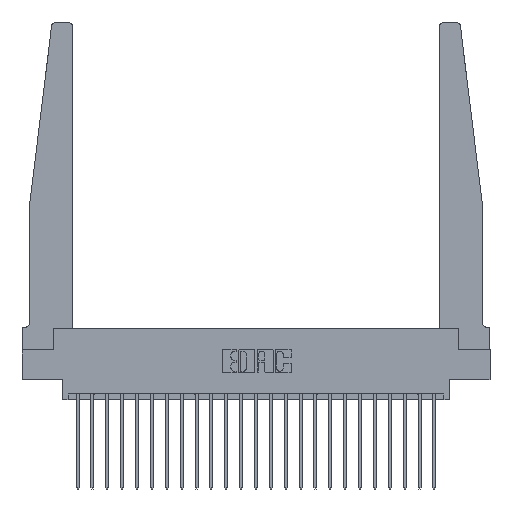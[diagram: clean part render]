
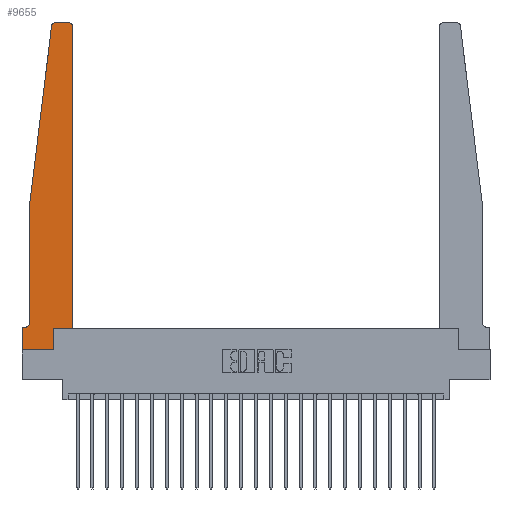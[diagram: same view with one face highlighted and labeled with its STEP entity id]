
A CAD part, top view. The second image highlights one B-rep face of the part: STEP entity #9655.
In plain terms, the highlighted planar face has unit normal (0, 0, 1).
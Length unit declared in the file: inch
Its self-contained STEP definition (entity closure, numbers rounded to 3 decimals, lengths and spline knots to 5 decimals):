
#130 = VERTEX_POINT ( 'NONE', #22104 ) ;
#207 = VERTEX_POINT ( 'NONE', #505 ) ;
#505 = CARTESIAN_POINT ( 'NONE',  ( 0.015, 0.1875, 0.37 ) ) ;
#706 = VERTEX_POINT ( 'NONE', #720 ) ;
#716 = CARTESIAN_POINT ( 'NONE',  ( 0., 0.1875, 0.37 ) ) ;
#720 = CARTESIAN_POINT ( 'NONE',  ( 0.2605, 0., 0.37 ) ) ;
#871 = DIRECTION ( 'NONE',  ( 0., 0., 1. ) ) ;
#1090 = EDGE_CURVE ( 'NONE', #130, #16308, #10998, .T. ) ;
#1507 = VERTEX_POINT ( 'NONE', #21269 ) ;
#1791 = DIRECTION ( 'NONE',  ( 0., 1., 0. ) ) ;
#1977 = CARTESIAN_POINT ( 'NONE',  ( 0.27653, 2.72, 0.37 ) ) ;
#2583 = CARTESIAN_POINT ( 'NONE',  ( 0.425, 0.18, 0.37 ) ) ;
#2689 = CARTESIAN_POINT ( 'NONE',  ( 0.065, 0.1875, 0.37 ) ) ;
#2743 = VERTEX_POINT ( 'NONE', #7454 ) ;
#2862 = ORIENTED_EDGE ( 'NONE', *, *, #20116, .T. ) ;
#3635 = CARTESIAN_POINT ( 'NONE',  ( 0.2605, 0.18, 0.37 ) ) ;
#3707 = DIRECTION ( 'NONE',  ( 0., -1., 0. ) ) ;
#3810 = CARTESIAN_POINT ( 'NONE',  ( 0.425, 2.72, 0.37 ) ) ;
#3836 = DIRECTION ( 'NONE',  ( 1., 0., 0. ) ) ;
#3937 = FACE_OUTER_BOUND ( 'NONE', #14693, .T. ) ;
#4645 = ORIENTED_EDGE ( 'NONE', *, *, #17247, .T. ) ;
#4728 = DIRECTION ( 'NONE',  ( -1., 0., 0. ) ) ;
#5217 = VECTOR ( 'NONE', #3707, 39.37008 ) ;
#5766 = LINE ( 'NONE', #12757, #5217 ) ;
#5909 = LINE ( 'NONE', #20548, #10140 ) ;
#6162 = CIRCLE ( 'NONE', #15299, 0.05 ) ;
#6211 = VECTOR ( 'NONE', #16327, 39.37008 ) ;
#6249 = DIRECTION ( 'NONE',  ( 0., 0., -1. ) ) ;
#6270 = CIRCLE ( 'NONE', #22259, 0.03 ) ;
#6960 = AXIS2_PLACEMENT_3D ( 'NONE', #1977, #14704, #3836 ) ;
#7123 = ORIENTED_EDGE ( 'NONE', *, *, #19761, .T. ) ;
#7146 = VECTOR ( 'NONE', #22930, 39.37008 ) ;
#7169 = LINE ( 'NONE', #10806, #16250 ) ;
#7206 = VECTOR ( 'NONE', #19050, 39.37008 ) ;
#7454 = CARTESIAN_POINT ( 'NONE',  ( 0.395, 2.75, 0.37 ) ) ;
#7500 = EDGE_CURVE ( 'NONE', #706, #10612, #20660, .T. ) ;
#7763 = LINE ( 'NONE', #2689, #7206 ) ;
#8116 = CARTESIAN_POINT ( 'NONE',  ( 0., 0.1875, 0.37 ) ) ;
#8241 = DIRECTION ( 'NONE',  ( 0., 0., 1. ) ) ;
#8249 = VECTOR ( 'NONE', #4728, 39.37008 ) ;
#9057 = ORIENTED_EDGE ( 'NONE', *, *, #22565, .T. ) ;
#9655 = ADVANCED_FACE ( 'NONE', ( #3937 ), #13528, .T. ) ;
#10140 = VECTOR ( 'NONE', #11482, 39.37008 ) ;
#10242 = EDGE_CURVE ( 'NONE', #16308, #11490, #5909, .T. ) ;
#10342 = ORIENTED_EDGE ( 'NONE', *, *, #7500, .T. ) ;
#10612 = VERTEX_POINT ( 'NONE', #10688 ) ;
#10688 = CARTESIAN_POINT ( 'NONE',  ( 0.2605, 0.18, 0.37 ) ) ;
#10806 = CARTESIAN_POINT ( 'NONE',  ( 0., 0., 0.37 ) ) ;
#10840 = CARTESIAN_POINT ( 'NONE',  ( 0.425, 0.18, 0.37 ) ) ;
#10980 = EDGE_CURVE ( 'NONE', #1507, #207, #6162, .T. ) ;
#10998 = CIRCLE ( 'NONE', #6960, 0.03 ) ;
#11482 = DIRECTION ( 'NONE',  ( -0.122, -0.992, 0. ) ) ;
#11490 = VERTEX_POINT ( 'NONE', #20161 ) ;
#12001 = VERTEX_POINT ( 'NONE', #3810 ) ;
#12338 = ORIENTED_EDGE ( 'NONE', *, *, #1090, .T. ) ;
#12711 = VECTOR ( 'NONE', #1791, 39.37008 ) ;
#12757 = CARTESIAN_POINT ( 'NONE',  ( 0.065, 1.25, 0.37 ) ) ;
#12985 = ORIENTED_EDGE ( 'NONE', *, *, #14779, .T. ) ;
#13301 = CARTESIAN_POINT ( 'NONE',  ( 0.24675, 2.72367, 0.37 ) ) ;
#13528 = PLANE ( 'NONE',  #19548 ) ;
#13613 = DIRECTION ( 'NONE',  ( 1., 0., 0. ) ) ;
#13623 = CARTESIAN_POINT ( 'NONE',  ( 0., 0., 0.37 ) ) ;
#13777 = CARTESIAN_POINT ( 'NONE',  ( 0.25, 2.75, 0.37 ) ) ;
#14084 = ORIENTED_EDGE ( 'NONE', *, *, #19326, .T. ) ;
#14602 = LINE ( 'NONE', #2583, #15749 ) ;
#14693 = EDGE_LOOP ( 'NONE', ( #12985, #12338, #22602, #2862, #23001, #7123, #23370, #20513, #10342, #14084, #4645, #9057 ) ) ;
#14704 = DIRECTION ( 'NONE',  ( 0., 0., 1. ) ) ;
#14779 = EDGE_CURVE ( 'NONE', #2743, #130, #22140, .T. ) ;
#15292 = DIRECTION ( 'NONE',  ( 1., 0., 0. ) ) ;
#15299 = AXIS2_PLACEMENT_3D ( 'NONE', #17094, #6249, #18932 ) ;
#15749 = VECTOR ( 'NONE', #15292, 39.37008 ) ;
#16250 = VECTOR ( 'NONE', #21757, 39.37008 ) ;
#16308 = VERTEX_POINT ( 'NONE', #13301 ) ;
#16327 = DIRECTION ( 'NONE',  ( 0., 1., 0. ) ) ;
#16779 = LINE ( 'NONE', #21112, #7146 ) ;
#17094 = CARTESIAN_POINT ( 'NONE',  ( 0.015, 0.2375, 0.37 ) ) ;
#17247 = EDGE_CURVE ( 'NONE', #21996, #12001, #22336, .T. ) ;
#18932 = DIRECTION ( 'NONE',  ( -1., 0., 0. ) ) ;
#19050 = DIRECTION ( 'NONE',  ( -1., 0., 0. ) ) ;
#19126 = CARTESIAN_POINT ( 'NONE',  ( 0.395, 2.72, 0.37 ) ) ;
#19326 = EDGE_CURVE ( 'NONE', #10612, #21996, #14602, .T. ) ;
#19548 = AXIS2_PLACEMENT_3D ( 'NONE', #8116, #871, #13613 ) ;
#19761 = EDGE_CURVE ( 'NONE', #207, #23206, #7763, .T. ) ;
#20116 = EDGE_CURVE ( 'NONE', #11490, #1507, #5766, .T. ) ;
#20161 = CARTESIAN_POINT ( 'NONE',  ( 0.065, 1.25, 0.37 ) ) ;
#20409 = VERTEX_POINT ( 'NONE', #13623 ) ;
#20513 = ORIENTED_EDGE ( 'NONE', *, *, #20740, .T. ) ;
#20548 = CARTESIAN_POINT ( 'NONE',  ( 0.065, 1.25, 0.37 ) ) ;
#20660 = LINE ( 'NONE', #3635, #6211 ) ;
#20740 = EDGE_CURVE ( 'NONE', #20409, #706, #7169, .T. ) ;
#20919 = DIRECTION ( 'NONE',  ( 1., 0., 0. ) ) ;
#21112 = CARTESIAN_POINT ( 'NONE',  ( 0., 0., 0.37 ) ) ;
#21176 = EDGE_CURVE ( 'NONE', #23206, #20409, #16779, .T. ) ;
#21269 = CARTESIAN_POINT ( 'NONE',  ( 0.065, 0.2375, 0.37 ) ) ;
#21712 = CARTESIAN_POINT ( 'NONE',  ( 0.425, 0.18, 0.37 ) ) ;
#21757 = DIRECTION ( 'NONE',  ( 1., 0., 0. ) ) ;
#21996 = VERTEX_POINT ( 'NONE', #21712 ) ;
#22104 = CARTESIAN_POINT ( 'NONE',  ( 0.27653, 2.75, 0.37 ) ) ;
#22140 = LINE ( 'NONE', #13777, #8249 ) ;
#22259 = AXIS2_PLACEMENT_3D ( 'NONE', #19126, #8241, #20919 ) ;
#22336 = LINE ( 'NONE', #10840, #12711 ) ;
#22565 = EDGE_CURVE ( 'NONE', #12001, #2743, #6270, .T. ) ;
#22602 = ORIENTED_EDGE ( 'NONE', *, *, #10242, .T. ) ;
#22930 = DIRECTION ( 'NONE',  ( 0., -1., 0. ) ) ;
#23001 = ORIENTED_EDGE ( 'NONE', *, *, #10980, .T. ) ;
#23206 = VERTEX_POINT ( 'NONE', #716 ) ;
#23370 = ORIENTED_EDGE ( 'NONE', *, *, #21176, .T. ) ;
